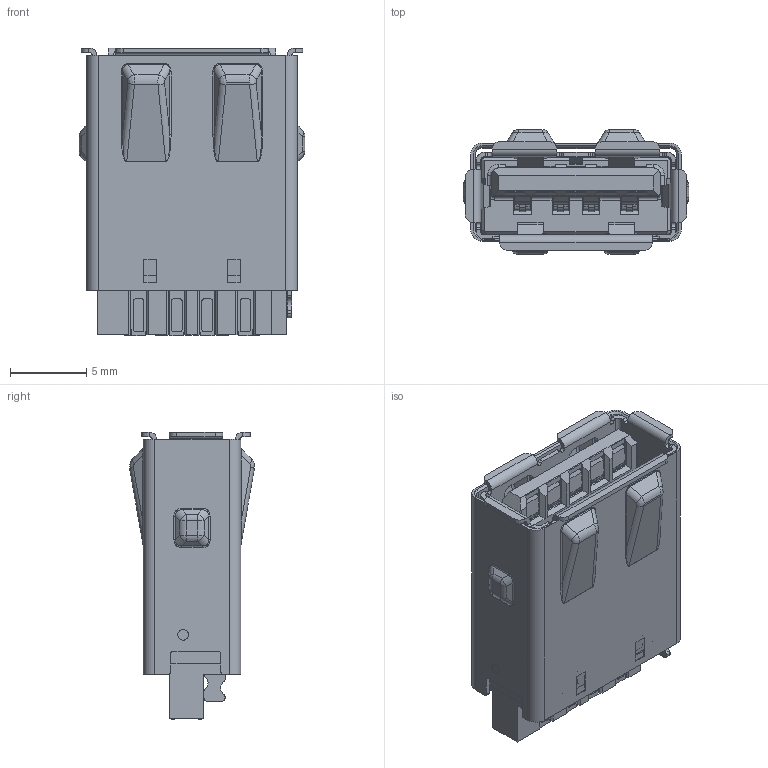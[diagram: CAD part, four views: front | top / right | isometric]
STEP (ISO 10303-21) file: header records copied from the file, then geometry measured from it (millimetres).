
FILE_DESCRIPTION (( 'STEP AP214' ), '1' );
FILE_NAME ('690M109J1AD-022.STEP', '2021-01-14T19:02:35', ( '' ), ( '' ), 'SwSTEP 2.0', 'SolidWorks 2020', '' );
FILE_SCHEMA (( 'AUTOMOTIVE_DESIGN' ));
Length unit declared in the file: millimetre
Products named in the file (10): 690M109J1AD-022; Contact2 690M109JXAD-02X; Contact1 690M109JXAD-02X; Contact5 3.0 690M109JXAD-02X; Contact3 690M109JXAD-02X; Contact4 690M109JXAD-02X; Jacket 690M109JXAD-02X; Shell 690M109JXAD-02X; Insulator2 690M109JXAD-02X_Blue; Insulator1 690M109JXAD-02X_Blue
Assembly tree (13 placements, depth 2):
  690M109J1AD-022
    Insulator1 690M109JXAD-02X_Blue
    Shell 690M109JXAD-02X
    Jacket 690M109JXAD-02X
    Contact5 3.0 690M109JXAD-02X  x5
    Contact1 690M109JXAD-02X
    Contact2 690M109JXAD-02X
    Contact3 690M109JXAD-02X
    Contact4 690M109JXAD-02X
    Insulator2 690M109JXAD-02X_Blue
Bounding box: 14.8 x 8.2 x 18.86 mm (x, y, z)
Volume: 810.7 mm3; surface area: 3982 mm2
Topology: 13 solids, 13 shells, 2416 faces, 6768 edges, 4355 vertices
Faces by surface type: plane 1451, cylinder 775, bspline 180, cone 10
Entity records: 67355 total; most frequent: CARTESIAN_POINT 15644, ORIENTED_EDGE 11232, DIRECTION 10138, EDGE_CURVE 5616, LINE 4132, VECTOR 4132, VERTEX_POINT 3619, AXIS2_PLACEMENT_3D 3003
